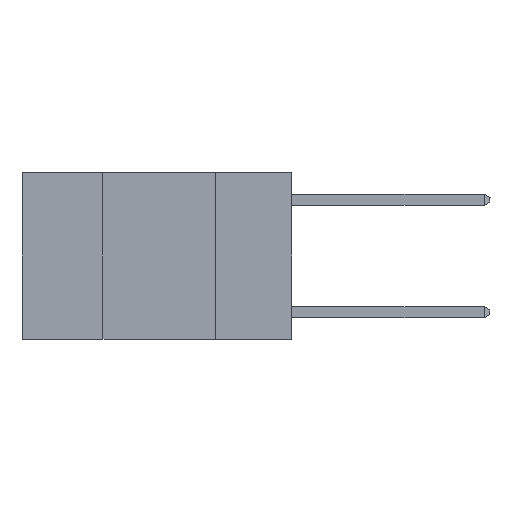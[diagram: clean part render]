
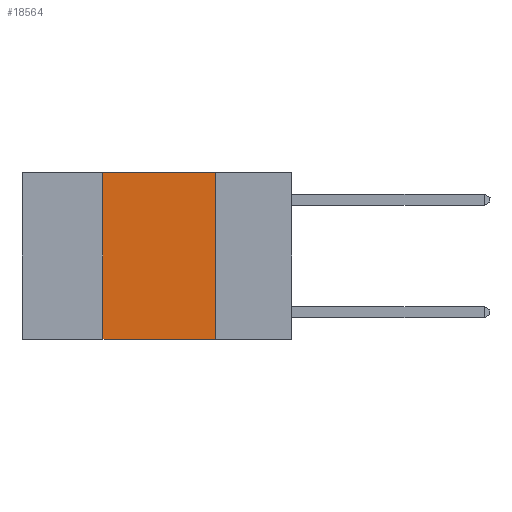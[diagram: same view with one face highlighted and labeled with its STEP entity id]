
A CAD part, left-side view. The second image highlights one B-rep face of the part: STEP entity #18564.
In plain terms, the highlighted planar face has unit normal (-1, 0, 0).
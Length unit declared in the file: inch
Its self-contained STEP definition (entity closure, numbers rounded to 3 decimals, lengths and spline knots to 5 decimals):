
#949 = VERTEX_POINT ( 'NONE', #4156 ) ;
#1066 = FACE_OUTER_BOUND ( 'NONE', #4101, .T. ) ;
#1485 = DIRECTION ( 'NONE',  ( 1., 0., 0. ) ) ;
#2261 = EDGE_CURVE ( 'NONE', #3649, #4209, #11645, .T. ) ;
#2285 = CARTESIAN_POINT ( 'NONE',  ( 0., 0.6, -0.37 ) ) ;
#2461 = EDGE_CURVE ( 'NONE', #949, #3649, #12403, .T. ) ;
#3141 = VERTEX_POINT ( 'NONE', #15631 ) ;
#3649 = VERTEX_POINT ( 'NONE', #17647 ) ;
#4101 = EDGE_LOOP ( 'NONE', ( #12443, #9268, #13961, #18497 ) ) ;
#4156 = CARTESIAN_POINT ( 'NONE',  ( 0., 0.42, -0.37 ) ) ;
#4209 = VERTEX_POINT ( 'NONE', #12547 ) ;
#4864 = EDGE_CURVE ( 'NONE', #949, #3141, #8683, .T. ) ;
#5268 = VECTOR ( 'NONE', #15971, 39.37008 ) ;
#5433 = CARTESIAN_POINT ( 'NONE',  ( 0., 0.6, 0. ) ) ;
#7008 = DIRECTION ( 'NONE',  ( 0., -1., 0. ) ) ;
#7490 = DIRECTION ( 'NONE',  ( 0., 0., -1. ) ) ;
#8411 = EDGE_CURVE ( 'NONE', #4209, #3141, #11646, .T. ) ;
#8683 = LINE ( 'NONE', #2285, #5268 ) ;
#9231 = VECTOR ( 'NONE', #9866, 39.37008 ) ;
#9268 = ORIENTED_EDGE ( 'NONE', *, *, #2261, .F. ) ;
#9866 = DIRECTION ( 'NONE',  ( 0., 0., -1. ) ) ;
#9957 = VECTOR ( 'NONE', #7008, 39.37008 ) ;
#11036 = CARTESIAN_POINT ( 'NONE',  ( 0., 0.42, 0. ) ) ;
#11645 = LINE ( 'NONE', #5433, #9957 ) ;
#11646 = LINE ( 'NONE', #12918, #9231 ) ;
#12175 = AXIS2_PLACEMENT_3D ( 'NONE', #14963, #1485, #7490 ) ;
#12403 = LINE ( 'NONE', #11036, #12767 ) ;
#12443 = ORIENTED_EDGE ( 'NONE', *, *, #8411, .F. ) ;
#12547 = CARTESIAN_POINT ( 'NONE',  ( 0., 0.17, 0. ) ) ;
#12767 = VECTOR ( 'NONE', #13972, 39.37008 ) ;
#12918 = CARTESIAN_POINT ( 'NONE',  ( 0., 0.17, 0. ) ) ;
#13961 = ORIENTED_EDGE ( 'NONE', *, *, #2461, .F. ) ;
#13972 = DIRECTION ( 'NONE',  ( 0., 0., 1. ) ) ;
#14963 = CARTESIAN_POINT ( 'NONE',  ( 0., 0.6, 0. ) ) ;
#15631 = CARTESIAN_POINT ( 'NONE',  ( 0., 0.17, -0.37 ) ) ;
#15971 = DIRECTION ( 'NONE',  ( 0., -1., 0. ) ) ;
#17647 = CARTESIAN_POINT ( 'NONE',  ( 0., 0.42, 0. ) ) ;
#18497 = ORIENTED_EDGE ( 'NONE', *, *, #4864, .T. ) ;
#18564 = ADVANCED_FACE ( 'NONE', ( #1066 ), #19390, .F. ) ;
#19390 = PLANE ( 'NONE',  #12175 ) ;
